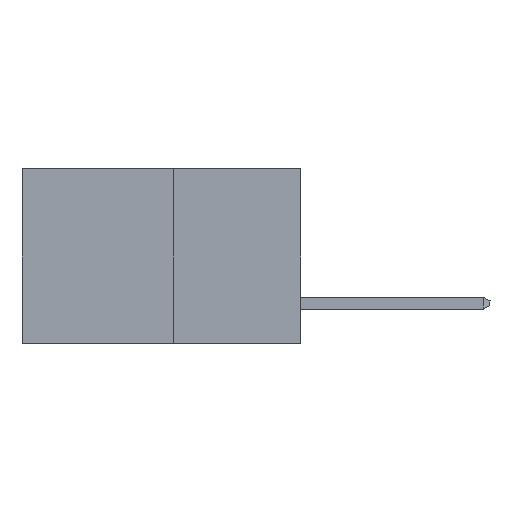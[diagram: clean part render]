
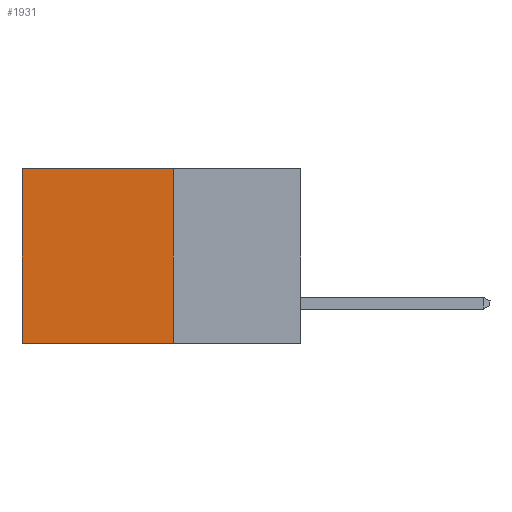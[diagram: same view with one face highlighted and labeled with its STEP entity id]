
A CAD part, left-side view. The second image highlights one B-rep face of the part: STEP entity #1931.
In plain terms, the highlighted planar face has unit normal (-1, 0, 0).
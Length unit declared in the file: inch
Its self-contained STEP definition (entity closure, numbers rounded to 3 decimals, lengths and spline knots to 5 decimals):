
#92 = VERTEX_POINT ( 'NONE', #13201 ) ;
#157 = VECTOR ( 'NONE', #2983, 39.37008 ) ;
#242 = PLANE ( 'NONE',  #1045 ) ;
#684 = EDGE_CURVE ( 'NONE', #92, #6140, #3290, .T. ) ;
#875 = CARTESIAN_POINT ( 'NONE',  ( 0.277, 0.27, -0.37 ) ) ;
#1045 = AXIS2_PLACEMENT_3D ( 'NONE', #875, #1841, #10049 ) ;
#1841 = DIRECTION ( 'NONE',  ( 1., 0., 0. ) ) ;
#1931 = ADVANCED_FACE ( 'NONE', ( #14869 ), #242, .F. ) ;
#1985 = ORIENTED_EDGE ( 'NONE', *, *, #13026, .T. ) ;
#2259 = CARTESIAN_POINT ( 'NONE',  ( 0.277, 0.59, -0.37 ) ) ;
#2983 = DIRECTION ( 'NONE',  ( 0., 0., -1. ) ) ;
#3290 = LINE ( 'NONE', #16474, #157 ) ;
#3388 = VECTOR ( 'NONE', #16119, 39.37008 ) ;
#3598 = DIRECTION ( 'NONE',  ( 0., 0., -1. ) ) ;
#4116 = CARTESIAN_POINT ( 'NONE',  ( 0.277, 0.59, -0.37 ) ) ;
#4413 = CARTESIAN_POINT ( 'NONE',  ( 0.277, 0.59, 0. ) ) ;
#4647 = VERTEX_POINT ( 'NONE', #4116 ) ;
#6140 = VERTEX_POINT ( 'NONE', #13061 ) ;
#6605 = VECTOR ( 'NONE', #15950, 39.37008 ) ;
#7102 = CARTESIAN_POINT ( 'NONE',  ( 0.277, 0.27, -0.37 ) ) ;
#7710 = LINE ( 'NONE', #2259, #13844 ) ;
#9373 = ORIENTED_EDGE ( 'NONE', *, *, #684, .F. ) ;
#10049 = DIRECTION ( 'NONE',  ( 0., 0., -1. ) ) ;
#10058 = LINE ( 'NONE', #10843, #6605 ) ;
#10843 = CARTESIAN_POINT ( 'NONE',  ( 0.277, 0.27, 0. ) ) ;
#12124 = ORIENTED_EDGE ( 'NONE', *, *, #16046, .T. ) ;
#12432 = VERTEX_POINT ( 'NONE', #4413 ) ;
#13026 = EDGE_CURVE ( 'NONE', #92, #12432, #10058, .T. ) ;
#13061 = CARTESIAN_POINT ( 'NONE',  ( 0.277, 0.27, -0.37 ) ) ;
#13201 = CARTESIAN_POINT ( 'NONE',  ( 0.277, 0.27, 0. ) ) ;
#13458 = LINE ( 'NONE', #7102, #3388 ) ;
#13844 = VECTOR ( 'NONE', #3598, 39.37008 ) ;
#14188 = EDGE_LOOP ( 'NONE', ( #12124, #16813, #9373, #1985 ) ) ;
#14869 = FACE_OUTER_BOUND ( 'NONE', #14188, .T. ) ;
#15950 = DIRECTION ( 'NONE',  ( 0., 1., 0. ) ) ;
#16046 = EDGE_CURVE ( 'NONE', #12432, #4647, #7710, .T. ) ;
#16119 = DIRECTION ( 'NONE',  ( 0., 1., 0. ) ) ;
#16474 = CARTESIAN_POINT ( 'NONE',  ( 0.277, 0.27, -0.37 ) ) ;
#16477 = EDGE_CURVE ( 'NONE', #6140, #4647, #13458, .T. ) ;
#16813 = ORIENTED_EDGE ( 'NONE', *, *, #16477, .F. ) ;
